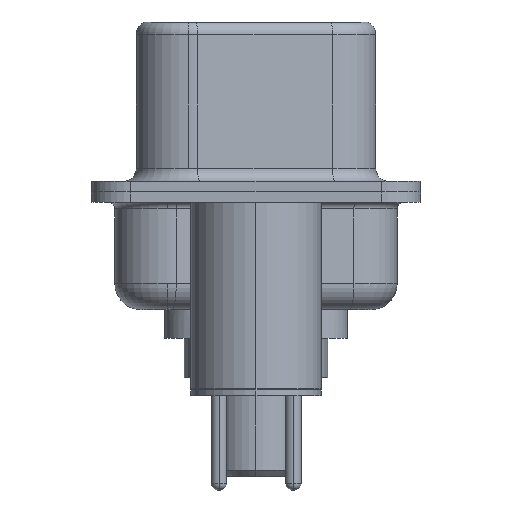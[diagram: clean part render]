
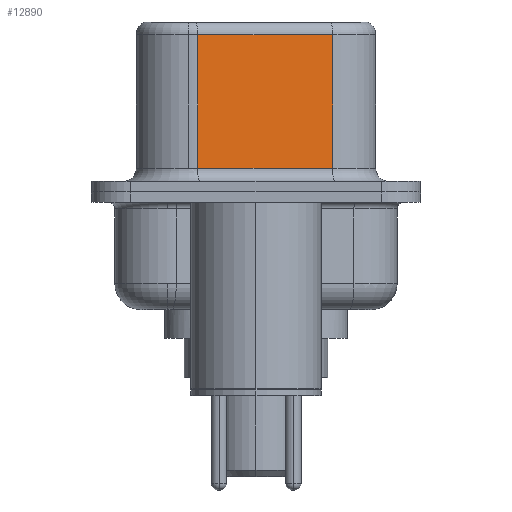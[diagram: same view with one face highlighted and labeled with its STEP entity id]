
A CAD part, left-side view. The second image highlights one B-rep face of the part: STEP entity #12890.
In plain terms, the highlighted planar face has unit normal (-0.985, -0.174, 0).
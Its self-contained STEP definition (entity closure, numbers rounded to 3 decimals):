
#42 = VECTOR ( 'NONE', #6344, 1000. ) ;
#69 = VECTOR ( 'NONE', #3396, 1000. ) ;
#371 = DIRECTION ( 'NONE',  ( -0.174, 0.985, 0. ) ) ;
#648 = LINE ( 'NONE', #9103, #12073 ) ;
#947 = CARTESIAN_POINT ( 'NONE',  ( 4.58, -2.927, 6.52 ) ) ;
#1167 = DIRECTION ( 'NONE',  ( -0.174, 0.985, 0. ) ) ;
#1658 = VERTEX_POINT ( 'NONE', #13916 ) ;
#1881 = DIRECTION ( 'NONE',  ( 0., 0., -1. ) ) ;
#2819 = VERTEX_POINT ( 'NONE', #7874 ) ;
#3396 = DIRECTION ( 'NONE',  ( 0., 0., -1. ) ) ;
#4462 = CARTESIAN_POINT ( 'NONE',  ( 3.67, 2.233, 6.52 ) ) ;
#5378 = VECTOR ( 'NONE', #1881, 1000. ) ;
#5914 = CARTESIAN_POINT ( 'NONE',  ( 3.67, 2.233, 0.9 ) ) ;
#6099 = PLANE ( 'NONE',  #12477 ) ;
#6323 = ORIENTED_EDGE ( 'NONE', *, *, #9339, .F. ) ;
#6344 = DIRECTION ( 'NONE',  ( 0.174, -0.985, 0. ) ) ;
#6367 = ORIENTED_EDGE ( 'NONE', *, *, #10326, .T. ) ;
#6387 = ORIENTED_EDGE ( 'NONE', *, *, #12025, .T. ) ;
#6581 = ORIENTED_EDGE ( 'NONE', *, *, #13574, .T. ) ;
#7188 = DIRECTION ( 'NONE',  ( 0.985, 0.174, 0. ) ) ;
#7874 = CARTESIAN_POINT ( 'NONE',  ( 4.58, -2.927, 0.9 ) ) ;
#9103 = CARTESIAN_POINT ( 'NONE',  ( 4.58, -2.927, 6.02 ) ) ;
#9333 = VERTEX_POINT ( 'NONE', #9645 ) ;
#9339 = EDGE_CURVE ( 'NONE', #9333, #2819, #11778, .T. ) ;
#9645 = CARTESIAN_POINT ( 'NONE',  ( 4.58, -2.927, 6.02 ) ) ;
#9733 = FACE_OUTER_BOUND ( 'NONE', #13575, .T. ) ;
#9931 = LINE ( 'NONE', #4462, #69 ) ;
#10326 = EDGE_CURVE ( 'NONE', #9333, #1658, #648, .T. ) ;
#10463 = VERTEX_POINT ( 'NONE', #5914 ) ;
#10950 = CARTESIAN_POINT ( 'NONE',  ( 4.58, -2.927, 0.9 ) ) ;
#11778 = LINE ( 'NONE', #947, #5378 ) ;
#12025 = EDGE_CURVE ( 'NONE', #1658, #10463, #9931, .T. ) ;
#12073 = VECTOR ( 'NONE', #1167, 1000. ) ;
#12157 = LINE ( 'NONE', #10950, #42 ) ;
#12477 = AXIS2_PLACEMENT_3D ( 'NONE', #13925, #7188, #371 ) ;
#12890 = ADVANCED_FACE ( 'NONE', ( #9733 ), #6099, .F. ) ;
#13574 = EDGE_CURVE ( 'NONE', #10463, #2819, #12157, .T. ) ;
#13575 = EDGE_LOOP ( 'NONE', ( #6323, #6367, #6387, #6581 ) ) ;
#13916 = CARTESIAN_POINT ( 'NONE',  ( 3.67, 2.233, 6.02 ) ) ;
#13925 = CARTESIAN_POINT ( 'NONE',  ( 4.58, -2.927, 6.52 ) ) ;
